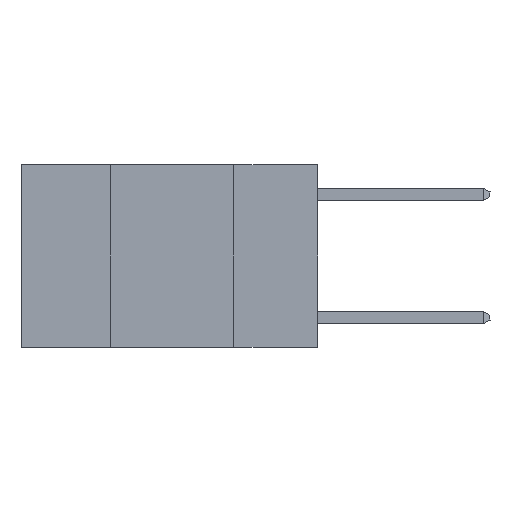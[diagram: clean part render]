
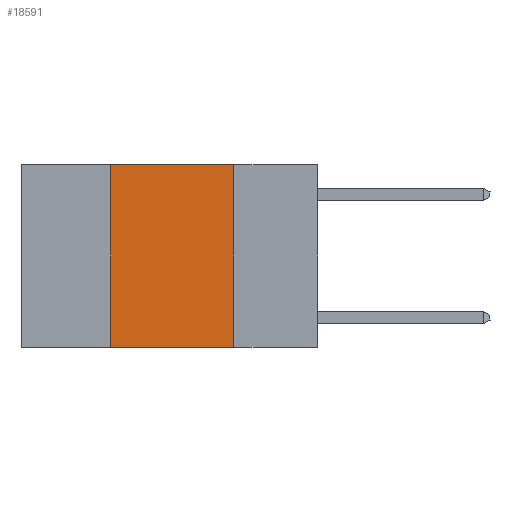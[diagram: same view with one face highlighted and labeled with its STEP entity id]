
A CAD part, left-side view. The second image highlights one B-rep face of the part: STEP entity #18591.
In plain terms, the highlighted planar face has unit normal (-1, 0, 0).
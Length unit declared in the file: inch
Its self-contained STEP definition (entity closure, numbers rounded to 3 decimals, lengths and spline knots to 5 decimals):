
#2052 = VECTOR ( 'NONE', #20361, 39.37008 ) ;
#2315 = CARTESIAN_POINT ( 'NONE',  ( 0., 0.6, 0. ) ) ;
#2556 = DIRECTION ( 'NONE',  ( 0., 0., -1. ) ) ;
#2833 = CARTESIAN_POINT ( 'NONE',  ( 0., 0.17, -0.37 ) ) ;
#2852 = ORIENTED_EDGE ( 'NONE', *, *, #11455, .F. ) ;
#3032 = DIRECTION ( 'NONE',  ( 0., -1., 0. ) ) ;
#3762 = EDGE_CURVE ( 'NONE', #16250, #9618, #13044, .T. ) ;
#4789 = PLANE ( 'NONE',  #19236 ) ;
#6363 = CARTESIAN_POINT ( 'NONE',  ( 0., 0.6, 0. ) ) ;
#8062 = ORIENTED_EDGE ( 'NONE', *, *, #15926, .F. ) ;
#8615 = LINE ( 'NONE', #6363, #23664 ) ;
#9618 = VERTEX_POINT ( 'NONE', #2833 ) ;
#11455 = EDGE_CURVE ( 'NONE', #21740, #14599, #8615, .T. ) ;
#13044 = LINE ( 'NONE', #18817, #24169 ) ;
#13936 = EDGE_LOOP ( 'NONE', ( #8062, #2852, #19878, #21790 ) ) ;
#14530 = FACE_OUTER_BOUND ( 'NONE', #13936, .T. ) ;
#14599 = VERTEX_POINT ( 'NONE', #14772 ) ;
#14772 = CARTESIAN_POINT ( 'NONE',  ( 0., 0.17, 0. ) ) ;
#15926 = EDGE_CURVE ( 'NONE', #14599, #9618, #16879, .T. ) ;
#16250 = VERTEX_POINT ( 'NONE', #22502 ) ;
#16363 = DIRECTION ( 'NONE',  ( 1., 0., 0. ) ) ;
#16879 = LINE ( 'NONE', #23198, #23320 ) ;
#18142 = LINE ( 'NONE', #20482, #2052 ) ;
#18591 = ADVANCED_FACE ( 'NONE', ( #14530 ), #4789, .F. ) ;
#18817 = CARTESIAN_POINT ( 'NONE',  ( 0., 0.6, -0.37 ) ) ;
#18862 = DIRECTION ( 'NONE',  ( 0., -1., 0. ) ) ;
#18874 = DIRECTION ( 'NONE',  ( 0., 0., -1. ) ) ;
#19236 = AXIS2_PLACEMENT_3D ( 'NONE', #2315, #16363, #18874 ) ;
#19878 = ORIENTED_EDGE ( 'NONE', *, *, #21278, .F. ) ;
#20361 = DIRECTION ( 'NONE',  ( 0., 0., 1. ) ) ;
#20482 = CARTESIAN_POINT ( 'NONE',  ( 0., 0.42, 0. ) ) ;
#21278 = EDGE_CURVE ( 'NONE', #16250, #21740, #18142, .T. ) ;
#21740 = VERTEX_POINT ( 'NONE', #22627 ) ;
#21790 = ORIENTED_EDGE ( 'NONE', *, *, #3762, .T. ) ;
#22502 = CARTESIAN_POINT ( 'NONE',  ( 0., 0.42, -0.37 ) ) ;
#22627 = CARTESIAN_POINT ( 'NONE',  ( 0., 0.42, 0. ) ) ;
#23198 = CARTESIAN_POINT ( 'NONE',  ( 0., 0.17, 0. ) ) ;
#23320 = VECTOR ( 'NONE', #2556, 39.37008 ) ;
#23664 = VECTOR ( 'NONE', #18862, 39.37008 ) ;
#24169 = VECTOR ( 'NONE', #3032, 39.37008 ) ;
